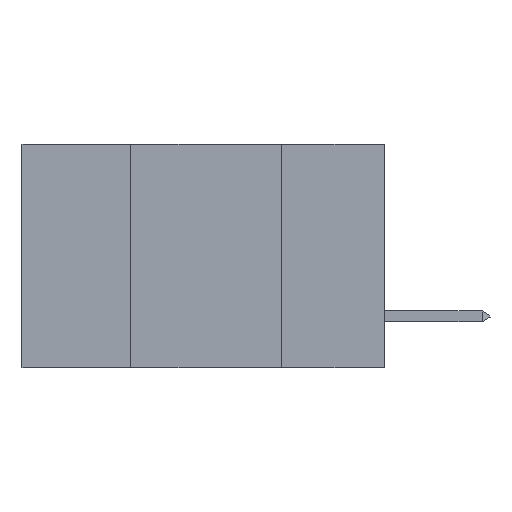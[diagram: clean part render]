
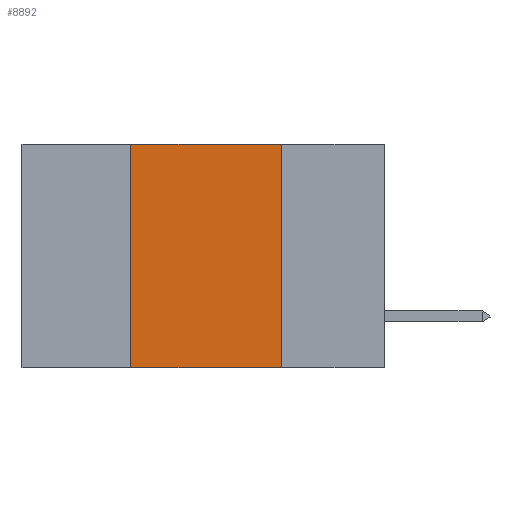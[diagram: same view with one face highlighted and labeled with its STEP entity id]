
A CAD part, left-side view. The second image highlights one B-rep face of the part: STEP entity #8892.
In plain terms, the highlighted planar face has unit normal (-1, 0, 0).
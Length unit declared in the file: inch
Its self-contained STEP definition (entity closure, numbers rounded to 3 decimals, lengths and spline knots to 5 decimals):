
#153 = LINE ( 'NONE', #11730, #4118 ) ;
#1572 = AXIS2_PLACEMENT_3D ( 'NONE', #13331, #9720, #14455 ) ;
#2359 = CARTESIAN_POINT ( 'NONE',  ( 0., 0.42, -0.37 ) ) ;
#2635 = VERTEX_POINT ( 'NONE', #7141 ) ;
#2911 = VECTOR ( 'NONE', #3015, 39.37008 ) ;
#3015 = DIRECTION ( 'NONE',  ( 0., -1., 0. ) ) ;
#3376 = ORIENTED_EDGE ( 'NONE', *, *, #10353, .F. ) ;
#4118 = VECTOR ( 'NONE', #13959, 39.37008 ) ;
#4264 = VECTOR ( 'NONE', #14886, 39.37008 ) ;
#4670 = DIRECTION ( 'NONE',  ( 0., 0., -1. ) ) ;
#5120 = CARTESIAN_POINT ( 'NONE',  ( 0., 0.17, 0. ) ) ;
#5220 = CARTESIAN_POINT ( 'NONE',  ( 0., 0.6, 0. ) ) ;
#5346 = ORIENTED_EDGE ( 'NONE', *, *, #13156, .F. ) ;
#6073 = LINE ( 'NONE', #11283, #4264 ) ;
#6274 = VECTOR ( 'NONE', #4670, 39.37008 ) ;
#6327 = VERTEX_POINT ( 'NONE', #5120 ) ;
#7032 = PLANE ( 'NONE',  #1572 ) ;
#7141 = CARTESIAN_POINT ( 'NONE',  ( 0., 0.17, -0.37 ) ) ;
#7516 = VERTEX_POINT ( 'NONE', #2359 ) ;
#7718 = EDGE_CURVE ( 'NONE', #7516, #2635, #6073, .T. ) ;
#8637 = FACE_OUTER_BOUND ( 'NONE', #12301, .T. ) ;
#8892 = ADVANCED_FACE ( 'NONE', ( #8637 ), #7032, .F. ) ;
#9479 = LINE ( 'NONE', #5220, #2911 ) ;
#9720 = DIRECTION ( 'NONE',  ( 1., 0., 0. ) ) ;
#10353 = EDGE_CURVE ( 'NONE', #14044, #6327, #9479, .T. ) ;
#11095 = LINE ( 'NONE', #12898, #6274 ) ;
#11283 = CARTESIAN_POINT ( 'NONE',  ( 0., 0.6, -0.37 ) ) ;
#11730 = CARTESIAN_POINT ( 'NONE',  ( 0., 0.42, 0. ) ) ;
#12065 = EDGE_CURVE ( 'NONE', #7516, #14044, #153, .T. ) ;
#12301 = EDGE_LOOP ( 'NONE', ( #5346, #3376, #13761, #14891 ) ) ;
#12898 = CARTESIAN_POINT ( 'NONE',  ( 0., 0.17, 0. ) ) ;
#13156 = EDGE_CURVE ( 'NONE', #6327, #2635, #11095, .T. ) ;
#13284 = CARTESIAN_POINT ( 'NONE',  ( 0., 0.42, 0. ) ) ;
#13331 = CARTESIAN_POINT ( 'NONE',  ( 0., 0.6, 0. ) ) ;
#13761 = ORIENTED_EDGE ( 'NONE', *, *, #12065, .F. ) ;
#13959 = DIRECTION ( 'NONE',  ( 0., 0., 1. ) ) ;
#14044 = VERTEX_POINT ( 'NONE', #13284 ) ;
#14455 = DIRECTION ( 'NONE',  ( 0., 0., -1. ) ) ;
#14886 = DIRECTION ( 'NONE',  ( 0., -1., 0. ) ) ;
#14891 = ORIENTED_EDGE ( 'NONE', *, *, #7718, .T. ) ;
